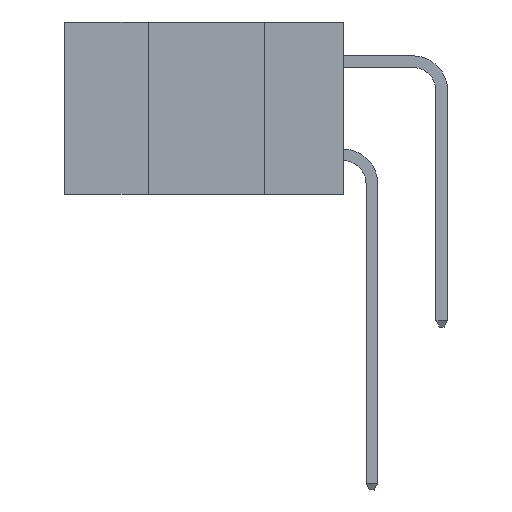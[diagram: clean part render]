
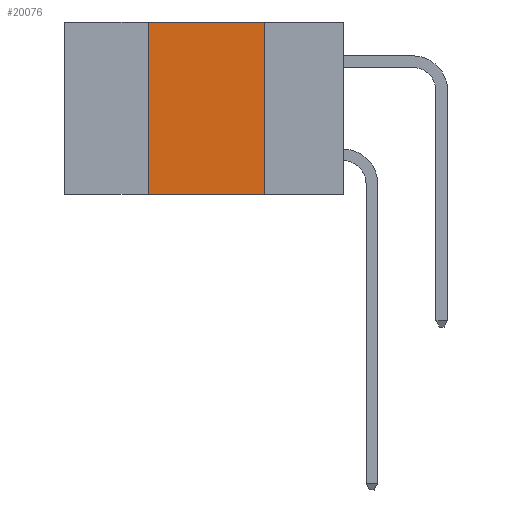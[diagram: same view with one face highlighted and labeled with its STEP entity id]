
A CAD part, left-side view. The second image highlights one B-rep face of the part: STEP entity #20076.
In plain terms, the highlighted planar face has unit normal (-1, 0, 0).
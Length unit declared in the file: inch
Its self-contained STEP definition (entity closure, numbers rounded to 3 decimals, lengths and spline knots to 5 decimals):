
#244 = CARTESIAN_POINT ( 'NONE',  ( 0., 0.42, -0.37 ) ) ;
#1965 = EDGE_CURVE ( 'NONE', #21022, #6139, #18469, .T. ) ;
#1972 = DIRECTION ( 'NONE',  ( 0., 0., -1. ) ) ;
#2042 = VECTOR ( 'NONE', #14330, 39.37008 ) ;
#2684 = CARTESIAN_POINT ( 'NONE',  ( 0., 0.6, 0. ) ) ;
#3219 = LINE ( 'NONE', #21557, #18945 ) ;
#4250 = DIRECTION ( 'NONE',  ( 0., -1., 0. ) ) ;
#6139 = VERTEX_POINT ( 'NONE', #20494 ) ;
#6801 = ORIENTED_EDGE ( 'NONE', *, *, #12344, .T. ) ;
#7199 = VECTOR ( 'NONE', #4250, 39.37008 ) ;
#7270 = CARTESIAN_POINT ( 'NONE',  ( 0., 0.42, 0. ) ) ;
#7495 = DIRECTION ( 'NONE',  ( 0., -1., 0. ) ) ;
#9025 = FACE_OUTER_BOUND ( 'NONE', #18237, .T. ) ;
#9443 = DIRECTION ( 'NONE',  ( 0., 0., -1. ) ) ;
#10329 = EDGE_CURVE ( 'NONE', #6139, #21471, #3219, .T. ) ;
#10880 = LINE ( 'NONE', #7270, #2042 ) ;
#11144 = CARTESIAN_POINT ( 'NONE',  ( 0., 0.6, 0. ) ) ;
#11905 = AXIS2_PLACEMENT_3D ( 'NONE', #11144, #19989, #9443 ) ;
#12344 = EDGE_CURVE ( 'NONE', #15406, #21471, #16138, .T. ) ;
#12391 = EDGE_CURVE ( 'NONE', #15406, #21022, #10880, .T. ) ;
#12768 = VECTOR ( 'NONE', #7495, 39.37008 ) ;
#14330 = DIRECTION ( 'NONE',  ( 0., 0., 1. ) ) ;
#15406 = VERTEX_POINT ( 'NONE', #244 ) ;
#16138 = LINE ( 'NONE', #16200, #12768 ) ;
#16200 = CARTESIAN_POINT ( 'NONE',  ( 0., 0.6, -0.37 ) ) ;
#17965 = ORIENTED_EDGE ( 'NONE', *, *, #10329, .F. ) ;
#18237 = EDGE_LOOP ( 'NONE', ( #17965, #21361, #18815, #6801 ) ) ;
#18406 = CARTESIAN_POINT ( 'NONE',  ( 0., 0.17, -0.37 ) ) ;
#18469 = LINE ( 'NONE', #2684, #7199 ) ;
#18815 = ORIENTED_EDGE ( 'NONE', *, *, #12391, .F. ) ;
#18945 = VECTOR ( 'NONE', #1972, 39.37008 ) ;
#19989 = DIRECTION ( 'NONE',  ( 1., 0., 0. ) ) ;
#20076 = ADVANCED_FACE ( 'NONE', ( #9025 ), #21698, .F. ) ;
#20494 = CARTESIAN_POINT ( 'NONE',  ( 0., 0.17, 0. ) ) ;
#21022 = VERTEX_POINT ( 'NONE', #22462 ) ;
#21361 = ORIENTED_EDGE ( 'NONE', *, *, #1965, .F. ) ;
#21471 = VERTEX_POINT ( 'NONE', #18406 ) ;
#21557 = CARTESIAN_POINT ( 'NONE',  ( 0., 0.17, 0. ) ) ;
#21698 = PLANE ( 'NONE',  #11905 ) ;
#22462 = CARTESIAN_POINT ( 'NONE',  ( 0., 0.42, 0. ) ) ;
